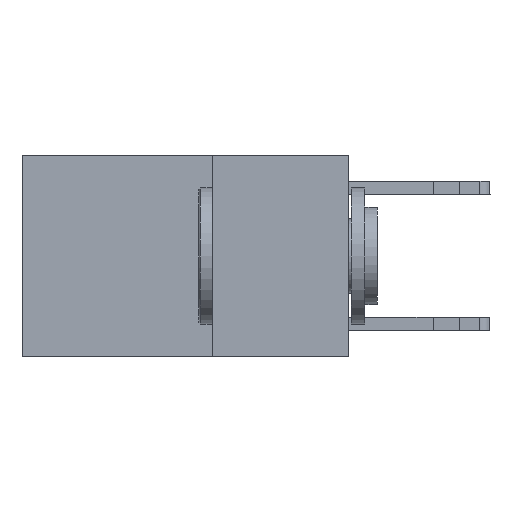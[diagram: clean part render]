
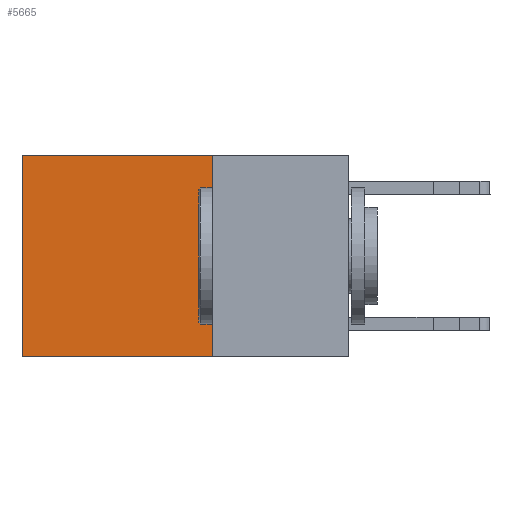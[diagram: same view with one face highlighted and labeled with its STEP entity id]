
A CAD part, left-side view. The second image highlights one B-rep face of the part: STEP entity #5665.
In plain terms, the highlighted planar face has unit normal (-1, 0, 0).
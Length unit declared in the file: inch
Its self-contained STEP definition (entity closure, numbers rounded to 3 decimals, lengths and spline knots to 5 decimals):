
#164 = LINE ( 'NONE', #5632, #1159 ) ;
#1159 = VECTOR ( 'NONE', #5162, 39.37008 ) ;
#2084 = CARTESIAN_POINT ( 'NONE',  ( 0.2625, 0.6, 0. ) ) ;
#2646 = PLANE ( 'NONE',  #14281 ) ;
#2725 = DIRECTION ( 'NONE',  ( 0., 0., -1. ) ) ;
#4321 = ORIENTED_EDGE ( 'NONE', *, *, #12084, .T. ) ;
#5162 = DIRECTION ( 'NONE',  ( 0., 0., -1. ) ) ;
#5632 = CARTESIAN_POINT ( 'NONE',  ( 0.2625, 0.6, 0. ) ) ;
#5665 = ADVANCED_FACE ( 'NONE', ( #12556 ), #2646, .F. ) ;
#5900 = LINE ( 'NONE', #10824, #12767 ) ;
#6782 = EDGE_CURVE ( 'NONE', #8163, #15240, #5900, .T. ) ;
#6808 = LINE ( 'NONE', #10141, #7696 ) ;
#7028 = LINE ( 'NONE', #8499, #15342 ) ;
#7547 = VERTEX_POINT ( 'NONE', #14107 ) ;
#7677 = EDGE_CURVE ( 'NONE', #7547, #8163, #7028, .T. ) ;
#7696 = VECTOR ( 'NONE', #15023, 39.37008 ) ;
#7947 = CARTESIAN_POINT ( 'NONE',  ( 0.2625, 0.25, 0. ) ) ;
#8163 = VERTEX_POINT ( 'NONE', #8639 ) ;
#8333 = DIRECTION ( 'NONE',  ( 0., 0., -1. ) ) ;
#8404 = ORIENTED_EDGE ( 'NONE', *, *, #11659, .T. ) ;
#8414 = VERTEX_POINT ( 'NONE', #2084 ) ;
#8499 = CARTESIAN_POINT ( 'NONE',  ( 0.2625, 0.25, 0. ) ) ;
#8639 = CARTESIAN_POINT ( 'NONE',  ( 0.2625, 0.25, -0.37 ) ) ;
#9920 = ORIENTED_EDGE ( 'NONE', *, *, #7677, .F. ) ;
#10141 = CARTESIAN_POINT ( 'NONE',  ( 0.2625, 0.25, 0. ) ) ;
#10567 = DIRECTION ( 'NONE',  ( 0., 1., 0. ) ) ;
#10752 = ORIENTED_EDGE ( 'NONE', *, *, #6782, .F. ) ;
#10824 = CARTESIAN_POINT ( 'NONE',  ( 0.2625, 0.25, -0.37 ) ) ;
#11659 = EDGE_CURVE ( 'NONE', #8414, #15240, #164, .T. ) ;
#12084 = EDGE_CURVE ( 'NONE', #7547, #8414, #6808, .T. ) ;
#12556 = FACE_OUTER_BOUND ( 'NONE', #15419, .T. ) ;
#12767 = VECTOR ( 'NONE', #10567, 39.37008 ) ;
#14083 = CARTESIAN_POINT ( 'NONE',  ( 0.2625, 0.6, -0.37 ) ) ;
#14107 = CARTESIAN_POINT ( 'NONE',  ( 0.2625, 0.25, 0. ) ) ;
#14281 = AXIS2_PLACEMENT_3D ( 'NONE', #7947, #15025, #2725 ) ;
#15023 = DIRECTION ( 'NONE',  ( 0., 1., 0. ) ) ;
#15025 = DIRECTION ( 'NONE',  ( 1., 0., 0. ) ) ;
#15240 = VERTEX_POINT ( 'NONE', #14083 ) ;
#15342 = VECTOR ( 'NONE', #8333, 39.37008 ) ;
#15419 = EDGE_LOOP ( 'NONE', ( #8404, #10752, #9920, #4321 ) ) ;
